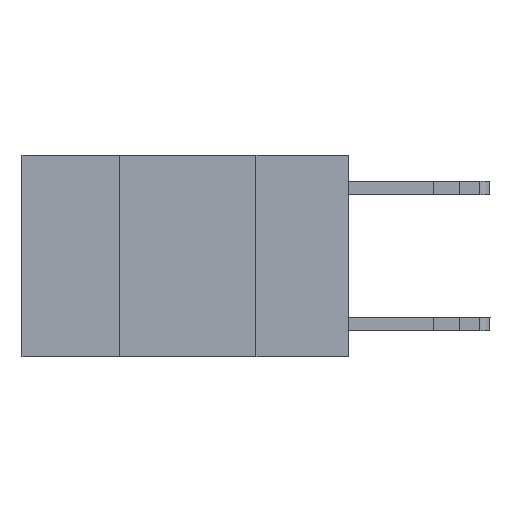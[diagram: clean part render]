
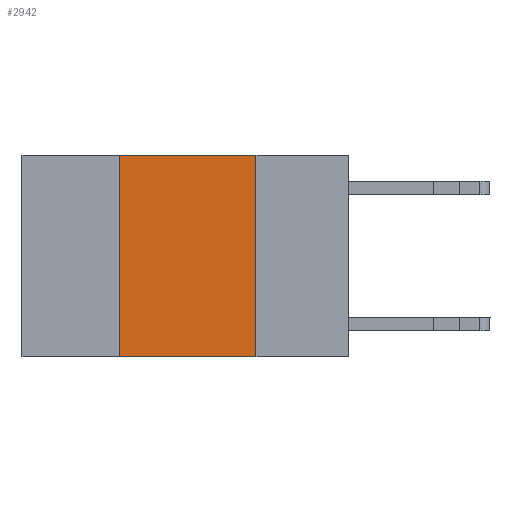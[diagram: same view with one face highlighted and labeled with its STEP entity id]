
A CAD part, left-side view. The second image highlights one B-rep face of the part: STEP entity #2942.
In plain terms, the highlighted planar face has unit normal (-1, 0, 0).
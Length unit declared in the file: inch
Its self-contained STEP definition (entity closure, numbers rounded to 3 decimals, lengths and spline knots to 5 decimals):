
#287 = CARTESIAN_POINT ( 'NONE',  ( 0., 0.42, 0. ) ) ;
#795 = EDGE_CURVE ( 'NONE', #9780, #3896, #10187, .T. ) ;
#1453 = ORIENTED_EDGE ( 'NONE', *, *, #22445, .F. ) ;
#1481 = DIRECTION ( 'NONE',  ( 0., 0., -1. ) ) ;
#1511 = DIRECTION ( 'NONE',  ( 1., 0., 0. ) ) ;
#1691 = CARTESIAN_POINT ( 'NONE',  ( 0., 0.6, 0. ) ) ;
#1719 = PLANE ( 'NONE',  #16097 ) ;
#2942 = ADVANCED_FACE ( 'NONE', ( #6165 ), #1719, .F. ) ;
#3896 = VERTEX_POINT ( 'NONE', #4911 ) ;
#4390 = CARTESIAN_POINT ( 'NONE',  ( 0., 0.6, -0.37 ) ) ;
#4911 = CARTESIAN_POINT ( 'NONE',  ( 0., 0.17, -0.37 ) ) ;
#5406 = ORIENTED_EDGE ( 'NONE', *, *, #21264, .T. ) ;
#5416 = CARTESIAN_POINT ( 'NONE',  ( 0., 0.42, -0.37 ) ) ;
#5582 = VECTOR ( 'NONE', #10334, 39.37008 ) ;
#5847 = LINE ( 'NONE', #8494, #5582 ) ;
#6009 = VERTEX_POINT ( 'NONE', #5416 ) ;
#6165 = FACE_OUTER_BOUND ( 'NONE', #7146, .T. ) ;
#6243 = DIRECTION ( 'NONE',  ( 0., -1., 0. ) ) ;
#6790 = DIRECTION ( 'NONE',  ( 0., 0., -1. ) ) ;
#7054 = CARTESIAN_POINT ( 'NONE',  ( 0., 0.17, 0. ) ) ;
#7146 = EDGE_LOOP ( 'NONE', ( #22379, #1453, #11404, #5406 ) ) ;
#8494 = CARTESIAN_POINT ( 'NONE',  ( 0., 0.6, 0. ) ) ;
#8588 = LINE ( 'NONE', #13164, #8701 ) ;
#8701 = VECTOR ( 'NONE', #9546, 39.37008 ) ;
#9546 = DIRECTION ( 'NONE',  ( 0., 0., 1. ) ) ;
#9778 = VECTOR ( 'NONE', #6790, 39.37008 ) ;
#9780 = VERTEX_POINT ( 'NONE', #16990 ) ;
#10187 = LINE ( 'NONE', #7054, #9778 ) ;
#10334 = DIRECTION ( 'NONE',  ( 0., -1., 0. ) ) ;
#11404 = ORIENTED_EDGE ( 'NONE', *, *, #22200, .F. ) ;
#13164 = CARTESIAN_POINT ( 'NONE',  ( 0., 0.42, 0. ) ) ;
#15035 = VERTEX_POINT ( 'NONE', #287 ) ;
#16097 = AXIS2_PLACEMENT_3D ( 'NONE', #1691, #1511, #1481 ) ;
#16990 = CARTESIAN_POINT ( 'NONE',  ( 0., 0.17, 0. ) ) ;
#19600 = VECTOR ( 'NONE', #6243, 39.37008 ) ;
#20090 = LINE ( 'NONE', #4390, #19600 ) ;
#21264 = EDGE_CURVE ( 'NONE', #6009, #3896, #20090, .T. ) ;
#22200 = EDGE_CURVE ( 'NONE', #6009, #15035, #8588, .T. ) ;
#22379 = ORIENTED_EDGE ( 'NONE', *, *, #795, .F. ) ;
#22445 = EDGE_CURVE ( 'NONE', #15035, #9780, #5847, .T. ) ;
